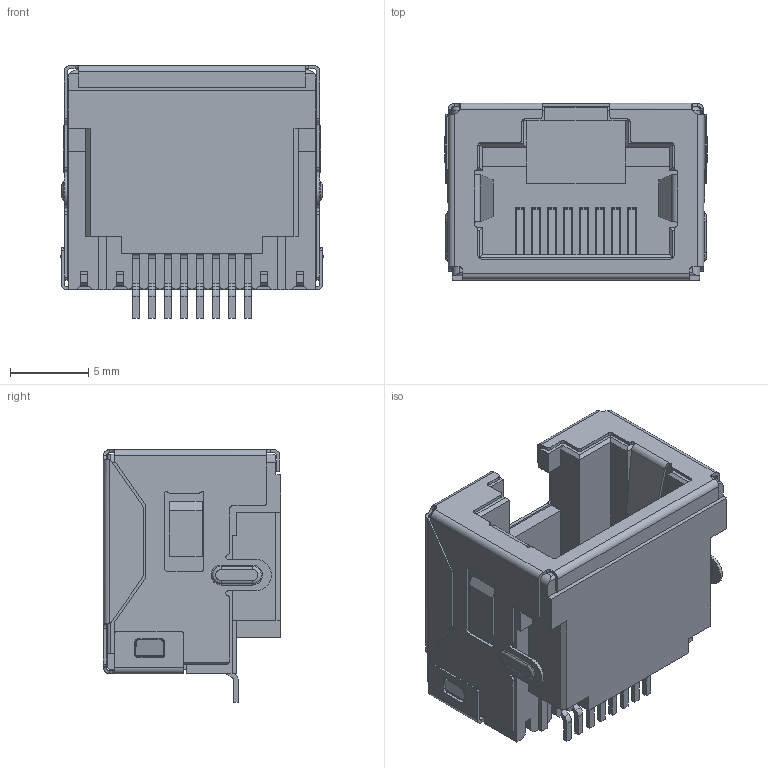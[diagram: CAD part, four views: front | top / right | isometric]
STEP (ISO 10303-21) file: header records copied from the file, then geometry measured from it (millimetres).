
FILE_DESCRIPTION (( 'STEP AP203' ), '1' );
FILE_NAME ('J6E018824N00110.STEP', '2020-03-19T13:18:02', ( '' ), ( '' ), 'SwSTEP 2.0', 'SolidWorks 2016', '' );
FILE_SCHEMA (( 'CONFIG_CONTROL_DESIGN' ));
Length unit declared in the file: millimetre
Products named in the file (4): 6E Shield_No LED; 6E Insulator_LED; 6E Contacts; J6E018824N00110
Assembly tree (3 placements, depth 2):
  J6E018824N00110
    6E Insulator_LED
    6E Contacts
    6E Shield_No LED
Bounding box: 16.75 x 11.3 x 16.12 mm (x, y, z)
Volume: 1065.3 mm3; surface area: 3845.6 mm2
Topology: 10 solids, 10 shells, 1430 faces, 4031 edges, 2610 vertices
Faces by surface type: plane 1053, cylinder 327, bspline 50
Entity records: 48105 total; most frequent: CARTESIAN_POINT 10763, ORIENTED_EDGE 8062, DIRECTION 7212, EDGE_CURVE 4031, LINE 3250, VECTOR 3250, VERTEX_POINT 2610, AXIS2_PLACEMENT_3D 1981
